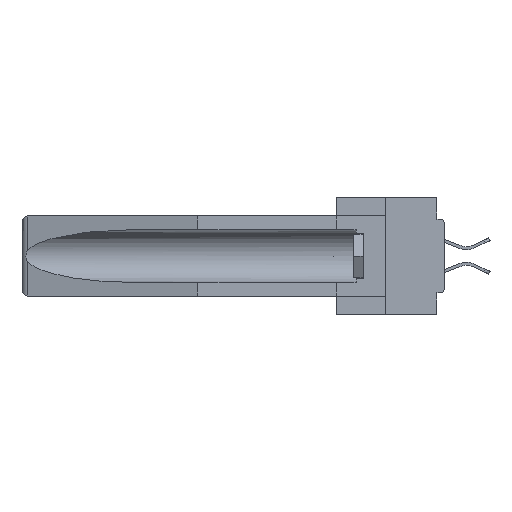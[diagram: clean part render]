
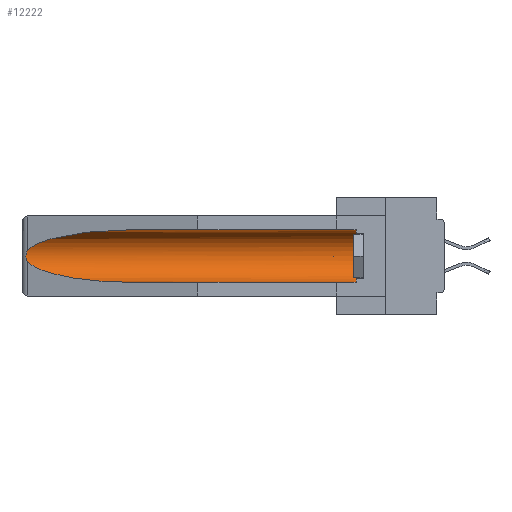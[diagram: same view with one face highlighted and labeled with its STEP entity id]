
A CAD part, left-side view. The second image highlights one B-rep face of the part: STEP entity #12222.
In plain terms, the highlighted cylindrical face has radius 2.857 mm (diameter 5.715 mm), a partial arc.
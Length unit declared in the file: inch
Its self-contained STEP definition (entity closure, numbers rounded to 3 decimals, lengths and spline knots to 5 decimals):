
#658 = CARTESIAN_POINT ( 'NONE',  ( 0.21114, 1.30732, -0.059 ) ) ;
#1136 = CARTESIAN_POINT ( 'NONE',  ( 0.155, 1.07973, -0.059 ) ) ;
#3200 = CARTESIAN_POINT ( 'NONE',  ( 0.26537, 1.52718, -0.19328 ) ) ;
#3628 = CARTESIAN_POINT ( 'NONE',  ( 0.26537, 1.52718, -0.14972 ) ) ;
#3930 = DIRECTION ( 'NONE',  ( 0., 1., 0. ) ) ;
#4923 = ORIENTED_EDGE ( 'NONE', *, *, #25381, .F. ) ;
#5148 = VERTEX_POINT ( 'NONE', #22889 ) ;
#8191 = VERTEX_POINT ( 'NONE', #3628 ) ;
#8738 = ORIENTED_EDGE ( 'NONE', *, *, #24128, .T. ) ;
#9770 = DIRECTION ( 'NONE',  ( 0., 1., 0. ) ) ;
#10095 = B_SPLINE_CURVE_WITH_KNOTS ( 'NONE', 3,
 ( #10409, #43720, #14159, #40347, #40495, #32705, #17868, #18193, #21447, #39867 ),
 .UNSPECIFIED., .F., .F.,
 ( 4, 2, 2, 2, 4 ),
 ( 0., 0.00029, 0.00058, 0.00087, 0.00117 ),
 .UNSPECIFIED. ) ;
#10242 = CIRCLE ( 'NONE', #35295, 0.1125 ) ;
#10409 = CARTESIAN_POINT ( 'NONE',  ( 0.26537, 1.52718, -0.14972 ) ) ;
#10698 =( BOUNDED_CURVE ( )  B_SPLINE_CURVE ( 3, ( #1136, #658, #27105, #11853 ),
 .UNSPECIFIED., .F., .F. ) 
 B_SPLINE_CURVE_WITH_KNOTS ( ( 4, 4 ),
 ( 4.71239, 6.08839 ),
 .UNSPECIFIED. ) 
 CURVE ( )  GEOMETRIC_REPRESENTATION_ITEM ( )  RATIONAL_B_SPLINE_CURVE ( ( 1., 0.848, 0.848, 1. ) ) 
 REPRESENTATION_ITEM ( '' )  );
#10820 = CARTESIAN_POINT ( 'NONE',  ( 0.155, 1.07973, -0.284 ) ) ;
#11351 = ORIENTED_EDGE ( 'NONE', *, *, #42235, .T. ) ;
#11469 = EDGE_CURVE ( 'NONE', #22928, #30908, #27990, .T. ) ;
#11571 = CARTESIAN_POINT ( 'NONE',  ( 0.155, -0.30754, -0.284 ) ) ;
#11853 = CARTESIAN_POINT ( 'NONE',  ( 0.26537, 1.52718, -0.14972 ) ) ;
#12222 = ADVANCED_FACE ( 'NONE', ( #32452 ), #13223, .F. ) ;
#12611 = DIRECTION ( 'NONE',  ( 0., -1., 0. ) ) ;
#13223 = CYLINDRICAL_SURFACE ( 'NONE', #29891, 0.1125 ) ;
#13598 = ORIENTED_EDGE ( 'NONE', *, *, #11469, .T. ) ;
#13973 = EDGE_LOOP ( 'NONE', ( #8738, #30875, #13598, #4923, #34669, #11351 ) ) ;
#14159 = CARTESIAN_POINT ( 'NONE',  ( 0.26654, 1.53092, -0.15636 ) ) ;
#16565 = EDGE_CURVE ( 'NONE', #21124, #5148, #10242, .T. ) ;
#17868 = CARTESIAN_POINT ( 'NONE',  ( 0.2673, 1.53269, -0.17917 ) ) ;
#18193 = CARTESIAN_POINT ( 'NONE',  ( 0.26655, 1.53094, -0.18657 ) ) ;
#19775 = DIRECTION ( 'NONE',  ( 0., 0., 1. ) ) ;
#20972 = EDGE_CURVE ( 'NONE', #8191, #22928, #10095, .T. ) ;
#21018 = CARTESIAN_POINT ( 'NONE',  ( 0.155, 1.07973, -0.059 ) ) ;
#21124 = VERTEX_POINT ( 'NONE', #40811 ) ;
#21288 = LINE ( 'NONE', #32072, #41642 ) ;
#21447 = CARTESIAN_POINT ( 'NONE',  ( 0.26597, 1.5296, -0.19026 ) ) ;
#22889 = CARTESIAN_POINT ( 'NONE',  ( 0.155, 0.126, -0.059 ) ) ;
#22928 = VERTEX_POINT ( 'NONE', #40984 ) ;
#24128 = EDGE_CURVE ( 'NONE', #35718, #8191, #10698, .T. ) ;
#25381 = EDGE_CURVE ( 'NONE', #21124, #30908, #42732, .T. ) ;
#27105 = CARTESIAN_POINT ( 'NONE',  ( 0.25451, 1.48313, -0.09465 ) ) ;
#27990 =( BOUNDED_CURVE ( )  B_SPLINE_CURVE ( 3, ( #3200, #29227, #36707, #10820 ),
 .UNSPECIFIED., .F., .T. ) 
 B_SPLINE_CURVE_WITH_KNOTS ( ( 4, 4 ),
 ( 0.1948, 1.5708 ),
 .UNSPECIFIED. ) 
 CURVE ( )  GEOMETRIC_REPRESENTATION_ITEM ( )  RATIONAL_B_SPLINE_CURVE ( ( 1., 0.848, 0.848, 1. ) ) 
 REPRESENTATION_ITEM ( '' )  );
#29063 = DIRECTION ( 'NONE',  ( 0., 0., 1. ) ) ;
#29227 = CARTESIAN_POINT ( 'NONE',  ( 0.25451, 1.48313, -0.24835 ) ) ;
#29891 = AXIS2_PLACEMENT_3D ( 'NONE', #36716, #36549, #29063 ) ;
#30875 = ORIENTED_EDGE ( 'NONE', *, *, #20972, .T. ) ;
#30908 = VERTEX_POINT ( 'NONE', #45733 ) ;
#31153 = CARTESIAN_POINT ( 'NONE',  ( 0.155, 0.126, -0.1715 ) ) ;
#32072 = CARTESIAN_POINT ( 'NONE',  ( 0.155, -0.30754, -0.059 ) ) ;
#32452 = FACE_OUTER_BOUND ( 'NONE', #13973, .T. ) ;
#32705 = CARTESIAN_POINT ( 'NONE',  ( 0.2675, 1.53308, -0.17534 ) ) ;
#34669 = ORIENTED_EDGE ( 'NONE', *, *, #16565, .T. ) ;
#35295 = AXIS2_PLACEMENT_3D ( 'NONE', #31153, #12611, #19775 ) ;
#35718 = VERTEX_POINT ( 'NONE', #21018 ) ;
#36549 = DIRECTION ( 'NONE',  ( 0., 1., 0. ) ) ;
#36707 = CARTESIAN_POINT ( 'NONE',  ( 0.21114, 1.30732, -0.284 ) ) ;
#36716 = CARTESIAN_POINT ( 'NONE',  ( 0.155, -0.30754, -0.1715 ) ) ;
#39867 = CARTESIAN_POINT ( 'NONE',  ( 0.26537, 1.52718, -0.19328 ) ) ;
#40347 = CARTESIAN_POINT ( 'NONE',  ( 0.2673, 1.5327, -0.16383 ) ) ;
#40495 = CARTESIAN_POINT ( 'NONE',  ( 0.2675, 1.53308, -0.16763 ) ) ;
#40811 = CARTESIAN_POINT ( 'NONE',  ( 0.155, 0.126, -0.284 ) ) ;
#40984 = CARTESIAN_POINT ( 'NONE',  ( 0.26537, 1.52718, -0.19328 ) ) ;
#41642 = VECTOR ( 'NONE', #9770, 39.37008 ) ;
#42235 = EDGE_CURVE ( 'NONE', #5148, #35718, #21288, .T. ) ;
#42732 = LINE ( 'NONE', #11571, #43890 ) ;
#43720 = CARTESIAN_POINT ( 'NONE',  ( 0.26597, 1.52961, -0.15275 ) ) ;
#43890 = VECTOR ( 'NONE', #3930, 39.37008 ) ;
#45733 = CARTESIAN_POINT ( 'NONE',  ( 0.155, 1.07973, -0.284 ) ) ;
